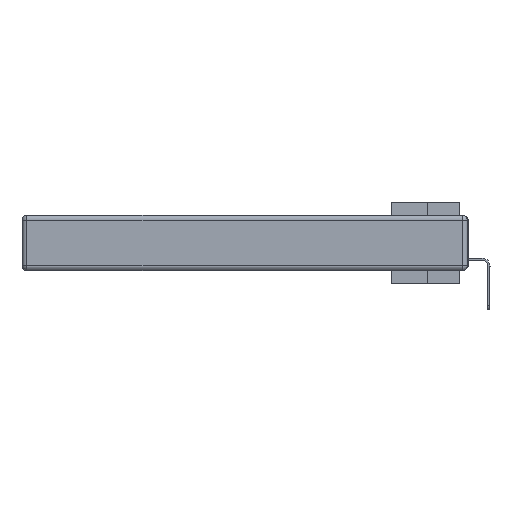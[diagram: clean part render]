
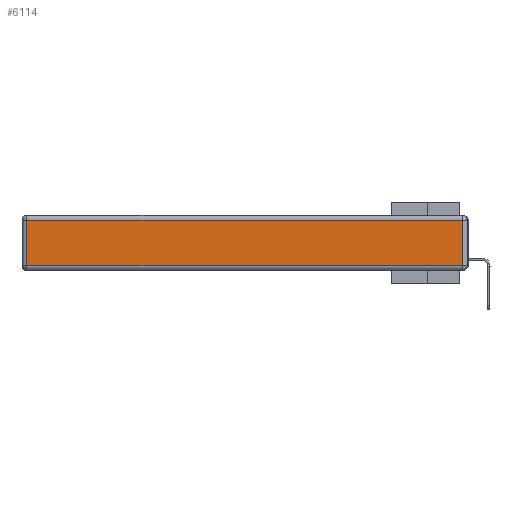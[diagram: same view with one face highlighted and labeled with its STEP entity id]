
A CAD part, left-side view. The second image highlights one B-rep face of the part: STEP entity #6114.
In plain terms, the highlighted planar face has unit normal (-1, 0, 0).
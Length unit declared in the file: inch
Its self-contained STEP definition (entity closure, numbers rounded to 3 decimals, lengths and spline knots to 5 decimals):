
#589 = CARTESIAN_POINT ( 'NONE',  ( 0., 0.03, -0.03 ) ) ;
#1214 = LINE ( 'NONE', #10627, #25355 ) ;
#1506 = DIRECTION ( 'NONE',  ( -1., 0., 0. ) ) ;
#3322 = AXIS2_PLACEMENT_3D ( 'NONE', #23935, #1506, #4236 ) ;
#4236 = DIRECTION ( 'NONE',  ( 0., 0., 1. ) ) ;
#4458 = PLANE ( 'NONE',  #3322 ) ;
#6114 = ADVANCED_FACE ( 'NONE', ( #31569 ), #4458, .T. ) ;
#6270 = CARTESIAN_POINT ( 'NONE',  ( 0., 0., -0.313 ) ) ;
#8524 = DIRECTION ( 'NONE',  ( 0., 0., -1. ) ) ;
#8833 = EDGE_CURVE ( 'NONE', #14787, #20857, #11178, .T. ) ;
#8915 = LINE ( 'NONE', #11532, #16692 ) ;
#9422 = CARTESIAN_POINT ( 'NONE',  ( 0., 2.72, -0.313 ) ) ;
#9807 = ORIENTED_EDGE ( 'NONE', *, *, #20190, .T. ) ;
#10627 = CARTESIAN_POINT ( 'NONE',  ( 0., 0.03, -0.343 ) ) ;
#11178 = LINE ( 'NONE', #16142, #13858 ) ;
#11532 = CARTESIAN_POINT ( 'NONE',  ( 0., 2.75, -0.03 ) ) ;
#13028 = ORIENTED_EDGE ( 'NONE', *, *, #31893, .T. ) ;
#13304 = CARTESIAN_POINT ( 'NONE',  ( 0., 0.03, -0.313 ) ) ;
#13585 = ORIENTED_EDGE ( 'NONE', *, *, #8833, .T. ) ;
#13858 = VECTOR ( 'NONE', #8524, 39.37008 ) ;
#14228 = DIRECTION ( 'NONE',  ( 0., 1., 0. ) ) ;
#14654 = EDGE_CURVE ( 'NONE', #30943, #25222, #1214, .T. ) ;
#14787 = VERTEX_POINT ( 'NONE', #18440 ) ;
#16142 = CARTESIAN_POINT ( 'NONE',  ( 0., 2.72, -0.343 ) ) ;
#16380 = DIRECTION ( 'NONE',  ( 0., -1., 0. ) ) ;
#16692 = VECTOR ( 'NONE', #14228, 39.37008 ) ;
#17938 = LINE ( 'NONE', #6270, #30387 ) ;
#18440 = CARTESIAN_POINT ( 'NONE',  ( 0., 2.72, -0.03 ) ) ;
#18665 = ORIENTED_EDGE ( 'NONE', *, *, #14654, .T. ) ;
#20190 = EDGE_CURVE ( 'NONE', #20857, #30943, #17938, .T. ) ;
#20857 = VERTEX_POINT ( 'NONE', #9422 ) ;
#23935 = CARTESIAN_POINT ( 'NONE',  ( 0., 0., -0.343 ) ) ;
#25222 = VERTEX_POINT ( 'NONE', #589 ) ;
#25355 = VECTOR ( 'NONE', #28027, 39.37008 ) ;
#28027 = DIRECTION ( 'NONE',  ( 0., 0., 1. ) ) ;
#28827 = EDGE_LOOP ( 'NONE', ( #9807, #18665, #13028, #13585 ) ) ;
#30387 = VECTOR ( 'NONE', #16380, 39.37008 ) ;
#30943 = VERTEX_POINT ( 'NONE', #13304 ) ;
#31569 = FACE_OUTER_BOUND ( 'NONE', #28827, .T. ) ;
#31893 = EDGE_CURVE ( 'NONE', #25222, #14787, #8915, .T. ) ;
